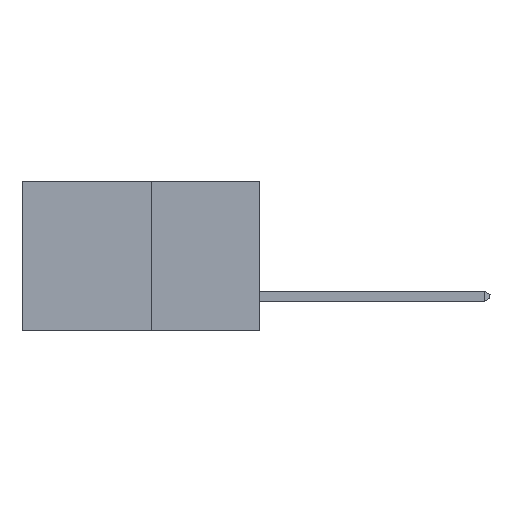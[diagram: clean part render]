
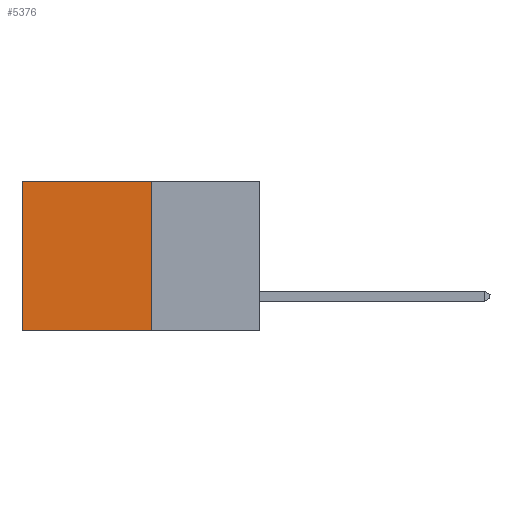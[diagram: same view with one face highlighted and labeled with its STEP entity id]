
A CAD part, left-side view. The second image highlights one B-rep face of the part: STEP entity #5376.
In plain terms, the highlighted planar face has unit normal (-1, 0, 0).
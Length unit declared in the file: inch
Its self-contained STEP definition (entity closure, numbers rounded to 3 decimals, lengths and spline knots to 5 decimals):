
#643 = ORIENTED_EDGE ( 'NONE', *, *, #9156, .T. ) ;
#1011 = DIRECTION ( 'NONE',  ( 0., 1., 0. ) ) ;
#1135 = CARTESIAN_POINT ( 'NONE',  ( 0.277, 0.59, -0.37 ) ) ;
#1560 = EDGE_CURVE ( 'NONE', #9691, #11703, #4865, .T. ) ;
#1954 = CARTESIAN_POINT ( 'NONE',  ( 0.277, 0.59, 0. ) ) ;
#2276 = VECTOR ( 'NONE', #3972, 39.37008 ) ;
#2671 = EDGE_CURVE ( 'NONE', #5958, #8315, #8384, .T. ) ;
#3215 = VECTOR ( 'NONE', #10959, 39.37008 ) ;
#3296 = CARTESIAN_POINT ( 'NONE',  ( 0.277, 0.27, 0. ) ) ;
#3972 = DIRECTION ( 'NONE',  ( 0., 0., -1. ) ) ;
#4159 = CARTESIAN_POINT ( 'NONE',  ( 0.277, 0.27, -0.37 ) ) ;
#4449 = CARTESIAN_POINT ( 'NONE',  ( 0.277, 0.27, 0. ) ) ;
#4697 = CARTESIAN_POINT ( 'NONE',  ( 0.277, 0.59, -0.37 ) ) ;
#4865 = LINE ( 'NONE', #1135, #13548 ) ;
#4933 = EDGE_LOOP ( 'NONE', ( #11200, #13980, #14311, #643 ) ) ;
#4962 = CARTESIAN_POINT ( 'NONE',  ( 0.277, 0.27, -0.37 ) ) ;
#4976 = LINE ( 'NONE', #4449, #11203 ) ;
#5308 = DIRECTION ( 'NONE',  ( 0., 0., -1. ) ) ;
#5345 = DIRECTION ( 'NONE',  ( 1., 0., 0. ) ) ;
#5376 = ADVANCED_FACE ( 'NONE', ( #7080 ), #5414, .F. ) ;
#5414 = PLANE ( 'NONE',  #8711 ) ;
#5958 = VERTEX_POINT ( 'NONE', #3296 ) ;
#7080 = FACE_OUTER_BOUND ( 'NONE', #4933, .T. ) ;
#8315 = VERTEX_POINT ( 'NONE', #10779 ) ;
#8384 = LINE ( 'NONE', #4159, #2276 ) ;
#8423 = EDGE_CURVE ( 'NONE', #8315, #11703, #12038, .T. ) ;
#8711 = AXIS2_PLACEMENT_3D ( 'NONE', #4962, #5345, #5308 ) ;
#8827 = CARTESIAN_POINT ( 'NONE',  ( 0.277, 0.27, -0.37 ) ) ;
#9156 = EDGE_CURVE ( 'NONE', #5958, #9691, #4976, .T. ) ;
#9691 = VERTEX_POINT ( 'NONE', #1954 ) ;
#10779 = CARTESIAN_POINT ( 'NONE',  ( 0.277, 0.27, -0.37 ) ) ;
#10959 = DIRECTION ( 'NONE',  ( 0., 1., 0. ) ) ;
#11200 = ORIENTED_EDGE ( 'NONE', *, *, #1560, .T. ) ;
#11203 = VECTOR ( 'NONE', #1011, 39.37008 ) ;
#11703 = VERTEX_POINT ( 'NONE', #4697 ) ;
#12038 = LINE ( 'NONE', #8827, #3215 ) ;
#12545 = DIRECTION ( 'NONE',  ( 0., 0., -1. ) ) ;
#13548 = VECTOR ( 'NONE', #12545, 39.37008 ) ;
#13980 = ORIENTED_EDGE ( 'NONE', *, *, #8423, .F. ) ;
#14311 = ORIENTED_EDGE ( 'NONE', *, *, #2671, .F. ) ;
